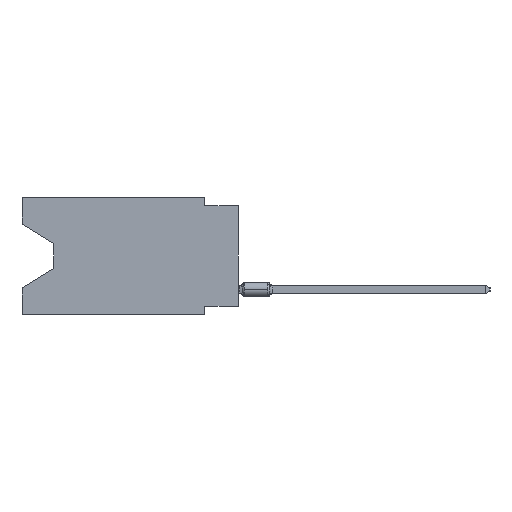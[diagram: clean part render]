
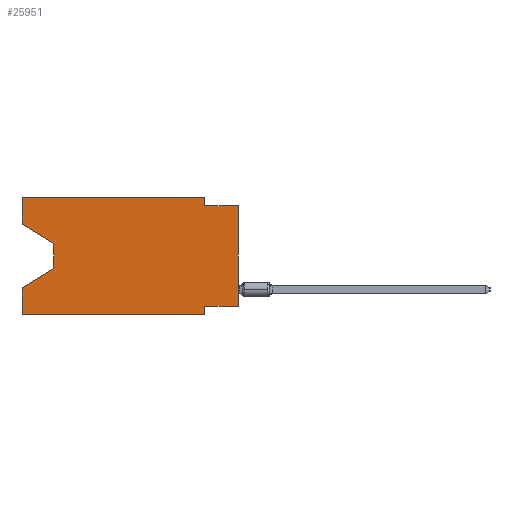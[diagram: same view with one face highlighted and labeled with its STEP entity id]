
A CAD part, left-side view. The second image highlights one B-rep face of the part: STEP entity #25951.
In plain terms, the highlighted planar face has unit normal (-1, 0, 0).
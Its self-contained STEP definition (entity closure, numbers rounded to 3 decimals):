
#25 = CARTESIAN_POINT ( 'NONE',  ( 0., 13.97, -3.505 ) ) ;
#150 = AXIS2_PLACEMENT_3D ( 'NONE', #42917, #8173, #9046 ) ;
#543 = CARTESIAN_POINT ( 'NONE',  ( 0., 0., 0. ) ) ;
#1047 = LINE ( 'NONE', #543, #8451 ) ;
#1400 = VERTEX_POINT ( 'NONE', #20023 ) ;
#1670 = CARTESIAN_POINT ( 'NONE',  ( 0., 16.383, -6.852 ) ) ;
#1949 = DIRECTION ( 'NONE',  ( 0., 0., 1. ) ) ;
#3893 = EDGE_LOOP ( 'NONE', ( #29281, #37507, #34115, #35206, #38628, #23206, #21195, #29761, #7389, #30004, #46239, #20487 ) ) ;
#4352 = CARTESIAN_POINT ( 'NONE',  ( 0., 13.97, -3.505 ) ) ;
#4444 = VERTEX_POINT ( 'NONE', #14531 ) ;
#4850 = VERTEX_POINT ( 'NONE', #41241 ) ;
#4856 = CARTESIAN_POINT ( 'NONE',  ( 0., 2.54, -0.635 ) ) ;
#4999 = EDGE_CURVE ( 'NONE', #4444, #10789, #1047, .T. ) ;
#5954 = CARTESIAN_POINT ( 'NONE',  ( 0., 2.54, -8.255 ) ) ;
#6043 = DIRECTION ( 'NONE',  ( 0., 0.855, -0.519 ) ) ;
#7389 = ORIENTED_EDGE ( 'NONE', *, *, #35854, .F. ) ;
#7421 = DIRECTION ( 'NONE',  ( 0., 0., -1. ) ) ;
#7652 = LINE ( 'NONE', #22547, #36459 ) ;
#8173 = DIRECTION ( 'NONE',  ( 1., 0., 0. ) ) ;
#8451 = VECTOR ( 'NONE', #45397, 1000. ) ;
#8732 = LINE ( 'NONE', #31154, #39684 ) ;
#8803 = CARTESIAN_POINT ( 'NONE',  ( 0., 16.383, 0. ) ) ;
#8962 = DIRECTION ( 'NONE',  ( 0., -1., 0. ) ) ;
#9046 = DIRECTION ( 'NONE',  ( 0., 0., -1. ) ) ;
#9937 = LINE ( 'NONE', #25097, #30523 ) ;
#10221 = CARTESIAN_POINT ( 'NONE',  ( 0., 16.383, 0. ) ) ;
#10631 = EDGE_CURVE ( 'NONE', #1400, #47129, #39696, .T. ) ;
#10789 = VERTEX_POINT ( 'NONE', #25577 ) ;
#11088 = LINE ( 'NONE', #43737, #36636 ) ;
#11220 = CARTESIAN_POINT ( 'NONE',  ( 0., 16.383, -8.89 ) ) ;
#12402 = DIRECTION ( 'NONE',  ( 0., 0., -1. ) ) ;
#13737 = DIRECTION ( 'NONE',  ( 0., -0.855, -0.519 ) ) ;
#14314 = EDGE_CURVE ( 'NONE', #28473, #27148, #46618, .T. ) ;
#14531 = CARTESIAN_POINT ( 'NONE',  ( 0., 0., -8.255 ) ) ;
#15234 = DIRECTION ( 'NONE',  ( 0., 0., -1. ) ) ;
#15859 = VECTOR ( 'NONE', #46297, 1000. ) ;
#17153 = VECTOR ( 'NONE', #13737, 1000. ) ;
#19069 = CARTESIAN_POINT ( 'NONE',  ( 0., 2.54, 0. ) ) ;
#19612 = VERTEX_POINT ( 'NONE', #4856 ) ;
#20023 = CARTESIAN_POINT ( 'NONE',  ( 0., 16.383, 0. ) ) ;
#20487 = ORIENTED_EDGE ( 'NONE', *, *, #32413, .F. ) ;
#20684 = CARTESIAN_POINT ( 'NONE',  ( 0., 16.383, 0. ) ) ;
#21195 = ORIENTED_EDGE ( 'NONE', *, *, #39692, .F. ) ;
#22424 = DIRECTION ( 'NONE',  ( 0., -1., 0. ) ) ;
#22547 = CARTESIAN_POINT ( 'NONE',  ( 0., 2.54, 0. ) ) ;
#23206 = ORIENTED_EDGE ( 'NONE', *, *, #42428, .F. ) ;
#23380 = VECTOR ( 'NONE', #12402, 1000. ) ;
#23586 = CARTESIAN_POINT ( 'NONE',  ( 0., 13.97, -5.385 ) ) ;
#24342 = LINE ( 'NONE', #20684, #37440 ) ;
#25097 = CARTESIAN_POINT ( 'NONE',  ( 0., 13.97, -5.385 ) ) ;
#25577 = CARTESIAN_POINT ( 'NONE',  ( 0., 0., -0.635 ) ) ;
#25600 = LINE ( 'NONE', #11220, #37266 ) ;
#25649 = CARTESIAN_POINT ( 'NONE',  ( 0., 0., -8.255 ) ) ;
#25951 = ADVANCED_FACE ( 'NONE', ( #37654 ), #31254, .F. ) ;
#26264 = VERTEX_POINT ( 'NONE', #1670 ) ;
#26412 = EDGE_CURVE ( 'NONE', #34027, #26264, #9937, .T. ) ;
#27148 = VERTEX_POINT ( 'NONE', #25 ) ;
#28024 = EDGE_CURVE ( 'NONE', #47129, #19612, #7652, .T. ) ;
#28473 = VERTEX_POINT ( 'NONE', #40250 ) ;
#28957 = EDGE_CURVE ( 'NONE', #48037, #4850, #25600, .T. ) ;
#29281 = ORIENTED_EDGE ( 'NONE', *, *, #14314, .T. ) ;
#29761 = ORIENTED_EDGE ( 'NONE', *, *, #4999, .T. ) ;
#30004 = ORIENTED_EDGE ( 'NONE', *, *, #28024, .F. ) ;
#30523 = VECTOR ( 'NONE', #6043, 1000. ) ;
#31154 = CARTESIAN_POINT ( 'NONE',  ( 0., 0., -0.635 ) ) ;
#31254 = PLANE ( 'NONE',  #150 ) ;
#32413 = EDGE_CURVE ( 'NONE', #28473, #1400, #45812, .T. ) ;
#34027 = VERTEX_POINT ( 'NONE', #23586 ) ;
#34115 = ORIENTED_EDGE ( 'NONE', *, *, #26412, .T. ) ;
#34381 = VECTOR ( 'NONE', #44863, 1000. ) ;
#34464 = CARTESIAN_POINT ( 'NONE',  ( 0., 16.383, -8.89 ) ) ;
#35206 = ORIENTED_EDGE ( 'NONE', *, *, #44175, .F. ) ;
#35854 = EDGE_CURVE ( 'NONE', #19612, #10789, #8732, .T. ) ;
#36459 = VECTOR ( 'NONE', #15234, 1000. ) ;
#36636 = VECTOR ( 'NONE', #7421, 1000. ) ;
#36852 = LINE ( 'NONE', #25649, #34381 ) ;
#37266 = VECTOR ( 'NONE', #22424, 1000. ) ;
#37440 = VECTOR ( 'NONE', #47415, 1000. ) ;
#37507 = ORIENTED_EDGE ( 'NONE', *, *, #37756, .T. ) ;
#37654 = FACE_OUTER_BOUND ( 'NONE', #3893, .T. ) ;
#37756 = EDGE_CURVE ( 'NONE', #27148, #34027, #45763, .T. ) ;
#38628 = ORIENTED_EDGE ( 'NONE', *, *, #28957, .T. ) ;
#38982 = VECTOR ( 'NONE', #1949, 1000. ) ;
#39684 = VECTOR ( 'NONE', #8962, 1000. ) ;
#39692 = EDGE_CURVE ( 'NONE', #4444, #42852, #36852, .T. ) ;
#39696 = LINE ( 'NONE', #10221, #15859 ) ;
#40250 = CARTESIAN_POINT ( 'NONE',  ( 0., 16.383, -2.038 ) ) ;
#41241 = CARTESIAN_POINT ( 'NONE',  ( 0., 2.54, -8.89 ) ) ;
#42428 = EDGE_CURVE ( 'NONE', #42852, #4850, #11088, .T. ) ;
#42852 = VERTEX_POINT ( 'NONE', #5954 ) ;
#42917 = CARTESIAN_POINT ( 'NONE',  ( 0., 16.383, 0. ) ) ;
#43737 = CARTESIAN_POINT ( 'NONE',  ( 0., 2.54, -8.89 ) ) ;
#44175 = EDGE_CURVE ( 'NONE', #48037, #26264, #24342, .T. ) ;
#44863 = DIRECTION ( 'NONE',  ( 0., 1., 0. ) ) ;
#45397 = DIRECTION ( 'NONE',  ( 0., 0., 1. ) ) ;
#45763 = LINE ( 'NONE', #4352, #23380 ) ;
#45812 = LINE ( 'NONE', #8803, #38982 ) ;
#46239 = ORIENTED_EDGE ( 'NONE', *, *, #10631, .F. ) ;
#46297 = DIRECTION ( 'NONE',  ( 0., -1., 0. ) ) ;
#46618 = LINE ( 'NONE', #47111, #17153 ) ;
#47111 = CARTESIAN_POINT ( 'NONE',  ( 0., 16.383, -2.038 ) ) ;
#47129 = VERTEX_POINT ( 'NONE', #19069 ) ;
#47415 = DIRECTION ( 'NONE',  ( 0., 0., 1. ) ) ;
#48037 = VERTEX_POINT ( 'NONE', #34464 ) ;
